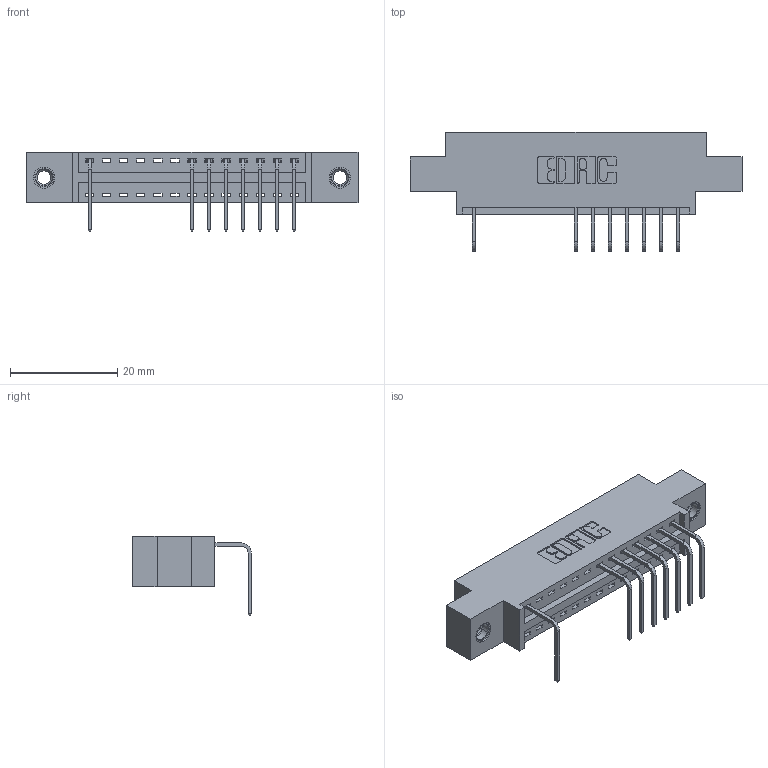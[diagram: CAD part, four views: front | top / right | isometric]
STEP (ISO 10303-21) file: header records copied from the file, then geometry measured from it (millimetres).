
FILE_DESCRIPTION (( 'STEP AP203' ), '1' );
FILE_NAME ('346-013-558-607.STEP', '2018-08-20T00:07:00', ( '' ), ( '' ), 'SwSTEP 2.0', 'SolidWorks 2016', '' );
FILE_SCHEMA (( 'CONFIG_CONTROL_DESIGN' ));
Length unit declared in the file: inch
Products named in the file (4): 345-292-001_558 Tail - 2; 345-250-001_345-250-005-103; 346-013-558-607; 346 Part_0.170 Offset - 0.156 Dia-TI
Assembly tree (11 placements, depth 2):
  346-013-558-607
    346 Part_0.170 Offset - 0.156 Dia-TI
    345-292-001_558 Tail - 2  x8
    345-250-001_345-250-005-103  x2
Bounding box: 61.85 x 22.16 x 14.73 mm (x, y, z)
Volume: 5521.9 mm3; surface area: 6635 mm2
Topology: 11 solids, 11 shells, 726 faces, 2143 edges, 1410 vertices
Faces by surface type: plane 498, cylinder 212, cone 12, torus 4
Entity records: 13214 total; most frequent: CARTESIAN_POINT 2281, ORIENTED_EDGE 2226, DIRECTION 2067, EDGE_CURVE 1113, VECTOR 909, LINE 909, VERTEX_POINT 736, AXIS2_PLACEMENT_3D 579
